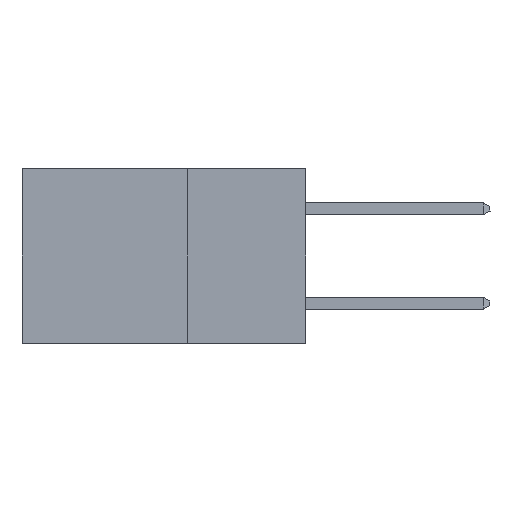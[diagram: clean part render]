
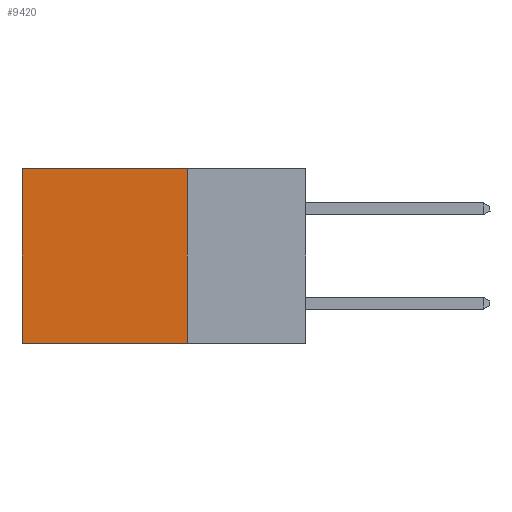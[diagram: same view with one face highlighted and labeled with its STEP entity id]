
A CAD part, left-side view. The second image highlights one B-rep face of the part: STEP entity #9420.
In plain terms, the highlighted planar face has unit normal (-1, 0, 0).
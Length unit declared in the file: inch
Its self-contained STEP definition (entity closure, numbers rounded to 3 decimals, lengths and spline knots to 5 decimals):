
#175 = EDGE_CURVE ( 'NONE', #9546, #8709, #9660, .T. ) ;
#515 = EDGE_CURVE ( 'NONE', #4404, #1471, #2648, .T. ) ;
#769 = ORIENTED_EDGE ( 'NONE', *, *, #515, .F. ) ;
#865 = CARTESIAN_POINT ( 'NONE',  ( 0.298, 0.6, 0. ) ) ;
#1006 = DIRECTION ( 'NONE',  ( 0., 1., 0. ) ) ;
#1045 = EDGE_CURVE ( 'NONE', #4404, #9546, #1101, .T. ) ;
#1101 = LINE ( 'NONE', #8293, #9503 ) ;
#1153 = CARTESIAN_POINT ( 'NONE',  ( 0.298, 0.25, -0.37 ) ) ;
#1364 = CARTESIAN_POINT ( 'NONE',  ( 0.298, 0.6, 0. ) ) ;
#1421 = DIRECTION ( 'NONE',  ( 0., 0., -1. ) ) ;
#1471 = VERTEX_POINT ( 'NONE', #5717 ) ;
#1528 = DIRECTION ( 'NONE',  ( 0., 0., -1. ) ) ;
#1638 = ORIENTED_EDGE ( 'NONE', *, *, #5920, .F. ) ;
#2335 = CARTESIAN_POINT ( 'NONE',  ( 0.298, 0.25, 0. ) ) ;
#2648 = LINE ( 'NONE', #6276, #10046 ) ;
#3635 = DIRECTION ( 'NONE',  ( 0., 1., 0. ) ) ;
#3845 = AXIS2_PLACEMENT_3D ( 'NONE', #2335, #5506, #1528 ) ;
#4404 = VERTEX_POINT ( 'NONE', #5345 ) ;
#4642 = DIRECTION ( 'NONE',  ( 0., 0., -1. ) ) ;
#5181 = FACE_OUTER_BOUND ( 'NONE', #6693, .T. ) ;
#5295 = ORIENTED_EDGE ( 'NONE', *, *, #175, .T. ) ;
#5345 = CARTESIAN_POINT ( 'NONE',  ( 0.298, 0.25, 0. ) ) ;
#5506 = DIRECTION ( 'NONE',  ( 1., 0., 0. ) ) ;
#5717 = CARTESIAN_POINT ( 'NONE',  ( 0.298, 0.25, -0.37 ) ) ;
#5920 = EDGE_CURVE ( 'NONE', #1471, #8709, #7156, .T. ) ;
#6199 = VECTOR ( 'NONE', #4642, 39.37008 ) ;
#6276 = CARTESIAN_POINT ( 'NONE',  ( 0.298, 0.25, 0. ) ) ;
#6693 = EDGE_LOOP ( 'NONE', ( #5295, #1638, #769, #7394 ) ) ;
#6776 = VECTOR ( 'NONE', #3635, 39.37008 ) ;
#7156 = LINE ( 'NONE', #1153, #6776 ) ;
#7394 = ORIENTED_EDGE ( 'NONE', *, *, #1045, .T. ) ;
#8293 = CARTESIAN_POINT ( 'NONE',  ( 0.298, 0.25, 0. ) ) ;
#8652 = CARTESIAN_POINT ( 'NONE',  ( 0.298, 0.6, -0.37 ) ) ;
#8709 = VERTEX_POINT ( 'NONE', #8652 ) ;
#9420 = ADVANCED_FACE ( 'NONE', ( #5181 ), #10383, .F. ) ;
#9503 = VECTOR ( 'NONE', #1006, 39.37008 ) ;
#9546 = VERTEX_POINT ( 'NONE', #865 ) ;
#9660 = LINE ( 'NONE', #1364, #6199 ) ;
#10046 = VECTOR ( 'NONE', #1421, 39.37008 ) ;
#10383 = PLANE ( 'NONE',  #3845 ) ;
